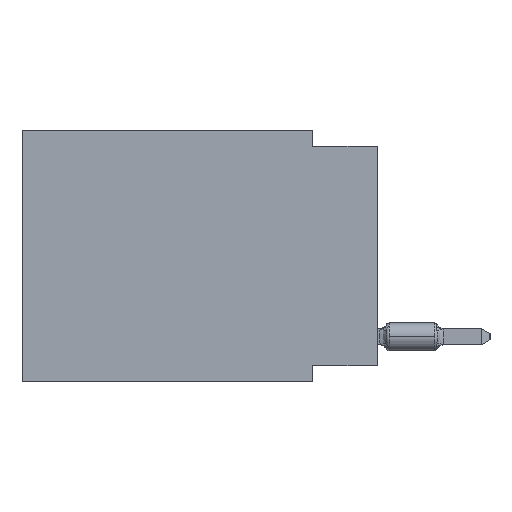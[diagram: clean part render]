
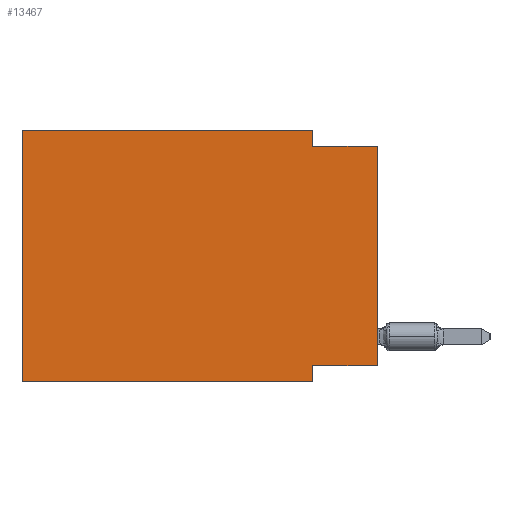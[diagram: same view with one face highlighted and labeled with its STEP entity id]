
A CAD part, left-side view. The second image highlights one B-rep face of the part: STEP entity #13467.
In plain terms, the highlighted planar face has unit normal (-1, 0, 0).
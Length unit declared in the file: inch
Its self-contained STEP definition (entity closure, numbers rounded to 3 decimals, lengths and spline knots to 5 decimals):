
#1102 = DIRECTION ( 'NONE',  ( 0., 0., -1. ) ) ;
#1500 = CARTESIAN_POINT ( 'NONE',  ( 0., 0.55, 0. ) ) ;
#2222 = CARTESIAN_POINT ( 'NONE',  ( 0., 0.55, 0. ) ) ;
#6055 = VECTOR ( 'NONE', #44170, 39.37008 ) ;
#6148 = DIRECTION ( 'NONE',  ( 0., 0., -1. ) ) ;
#6986 = DIRECTION ( 'NONE',  ( 0., -1., 0. ) ) ;
#7446 = EDGE_CURVE ( 'NONE', #16279, #27871, #60445, .T. ) ;
#7985 = EDGE_LOOP ( 'NONE', ( #54028, #18264, #21485, #68171, #52991, #56376, #30633, #17442 ) ) ;
#8010 = VERTEX_POINT ( 'NONE', #47822 ) ;
#8504 = CARTESIAN_POINT ( 'NONE',  ( 0., 0., -0.365 ) ) ;
#8703 = VERTEX_POINT ( 'NONE', #56253 ) ;
#9136 = CARTESIAN_POINT ( 'NONE',  ( 0., 0., -0.025 ) ) ;
#9804 = VECTOR ( 'NONE', #6148, 39.37008 ) ;
#10880 = VERTEX_POINT ( 'NONE', #69152 ) ;
#11389 = LINE ( 'NONE', #49096, #15415 ) ;
#12458 = VECTOR ( 'NONE', #22444, 39.37008 ) ;
#13467 = ADVANCED_FACE ( 'NONE', ( #62321 ), #45574, .F. ) ;
#13726 = EDGE_CURVE ( 'NONE', #27871, #10880, #11389, .T. ) ;
#15415 = VECTOR ( 'NONE', #1102, 39.37008 ) ;
#16258 = CARTESIAN_POINT ( 'NONE',  ( 0., 0.55, -0.39 ) ) ;
#16279 = VERTEX_POINT ( 'NONE', #8504 ) ;
#17442 = ORIENTED_EDGE ( 'NONE', *, *, #7446, .F. ) ;
#17846 = DIRECTION ( 'NONE',  ( 0., 0., -1. ) ) ;
#18264 = ORIENTED_EDGE ( 'NONE', *, *, #22846, .F. ) ;
#20871 = LINE ( 'NONE', #42584, #69649 ) ;
#21485 = ORIENTED_EDGE ( 'NONE', *, *, #35918, .F. ) ;
#22082 = VECTOR ( 'NONE', #6986, 39.37008 ) ;
#22444 = DIRECTION ( 'NONE',  ( 0., 0., 1. ) ) ;
#22846 = EDGE_CURVE ( 'NONE', #8010, #45629, #20871, .T. ) ;
#23513 = LINE ( 'NONE', #1500, #6055 ) ;
#24071 = DIRECTION ( 'NONE',  ( 0., 1., 0. ) ) ;
#26217 = LINE ( 'NONE', #16258, #45621 ) ;
#27467 = CARTESIAN_POINT ( 'NONE',  ( 0., 0.1, 0. ) ) ;
#27871 = VERTEX_POINT ( 'NONE', #48856 ) ;
#29905 = EDGE_CURVE ( 'NONE', #64955, #8703, #23513, .T. ) ;
#30633 = ORIENTED_EDGE ( 'NONE', *, *, #13726, .F. ) ;
#34206 = CARTESIAN_POINT ( 'NONE',  ( 0., 0.1, 0. ) ) ;
#34891 = DIRECTION ( 'NONE',  ( 1., 0., 0. ) ) ;
#35789 = CARTESIAN_POINT ( 'NONE',  ( 0., 0., -0.365 ) ) ;
#35918 = EDGE_CURVE ( 'NONE', #51122, #8010, #65566, .T. ) ;
#37404 = CARTESIAN_POINT ( 'NONE',  ( 0., 0., 0. ) ) ;
#42106 = EDGE_CURVE ( 'NONE', #16279, #45629, #54168, .T. ) ;
#42216 = DIRECTION ( 'NONE',  ( 0., -1., 0. ) ) ;
#42584 = CARTESIAN_POINT ( 'NONE',  ( 0., 0., -0.025 ) ) ;
#44170 = DIRECTION ( 'NONE',  ( 0., 0., 1. ) ) ;
#45574 = PLANE ( 'NONE',  #59764 ) ;
#45621 = VECTOR ( 'NONE', #42216, 39.37008 ) ;
#45629 = VERTEX_POINT ( 'NONE', #9136 ) ;
#47822 = CARTESIAN_POINT ( 'NONE',  ( 0., 0.1, -0.025 ) ) ;
#48856 = CARTESIAN_POINT ( 'NONE',  ( 0., 0.1, -0.365 ) ) ;
#48977 = CARTESIAN_POINT ( 'NONE',  ( 0., 0.55, 0. ) ) ;
#49096 = CARTESIAN_POINT ( 'NONE',  ( 0., 0.1, -0.39 ) ) ;
#49330 = LINE ( 'NONE', #48977, #22082 ) ;
#51122 = VERTEX_POINT ( 'NONE', #34206 ) ;
#52991 = ORIENTED_EDGE ( 'NONE', *, *, #29905, .F. ) ;
#54028 = ORIENTED_EDGE ( 'NONE', *, *, #42106, .T. ) ;
#54168 = LINE ( 'NONE', #37404, #12458 ) ;
#55239 = EDGE_CURVE ( 'NONE', #64955, #10880, #26217, .T. ) ;
#56253 = CARTESIAN_POINT ( 'NONE',  ( 0., 0.55, 0. ) ) ;
#56376 = ORIENTED_EDGE ( 'NONE', *, *, #55239, .T. ) ;
#59764 = AXIS2_PLACEMENT_3D ( 'NONE', #2222, #34891, #17846 ) ;
#60445 = LINE ( 'NONE', #35789, #63182 ) ;
#60668 = EDGE_CURVE ( 'NONE', #8703, #51122, #49330, .T. ) ;
#62321 = FACE_OUTER_BOUND ( 'NONE', #7985, .T. ) ;
#63182 = VECTOR ( 'NONE', #24071, 39.37008 ) ;
#64327 = DIRECTION ( 'NONE',  ( 0., -1., 0. ) ) ;
#64955 = VERTEX_POINT ( 'NONE', #66601 ) ;
#65566 = LINE ( 'NONE', #27467, #9804 ) ;
#66601 = CARTESIAN_POINT ( 'NONE',  ( 0., 0.55, -0.39 ) ) ;
#68171 = ORIENTED_EDGE ( 'NONE', *, *, #60668, .F. ) ;
#69152 = CARTESIAN_POINT ( 'NONE',  ( 0., 0.1, -0.39 ) ) ;
#69649 = VECTOR ( 'NONE', #64327, 39.37008 ) ;
